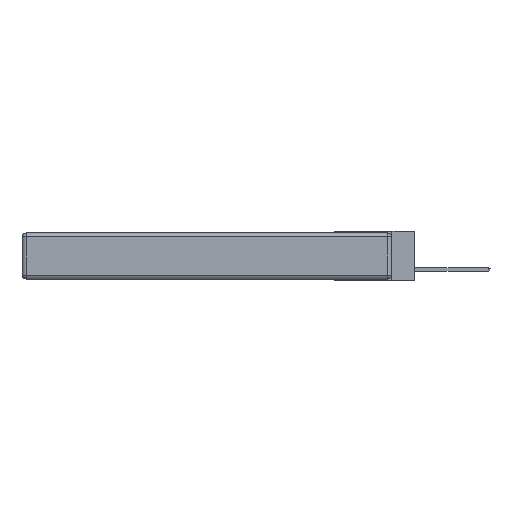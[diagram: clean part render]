
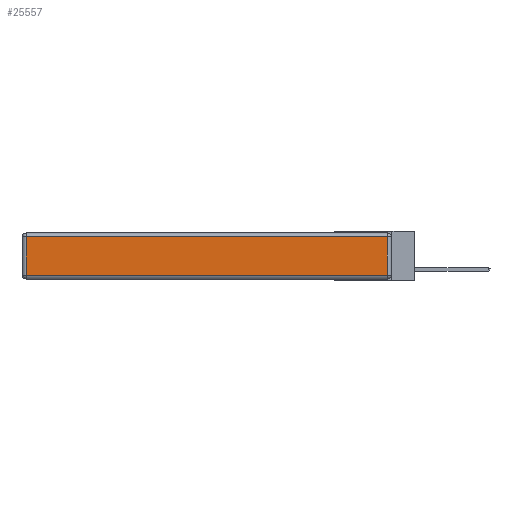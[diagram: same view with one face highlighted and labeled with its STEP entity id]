
A CAD part, left-side view. The second image highlights one B-rep face of the part: STEP entity #25557.
In plain terms, the highlighted planar face has unit normal (-1, 0, 0).
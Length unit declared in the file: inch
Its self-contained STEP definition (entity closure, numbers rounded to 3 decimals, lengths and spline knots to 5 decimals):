
#193 = AXIS2_PLACEMENT_3D ( 'NONE', #6007, #12641, #1880 ) ;
#812 = CARTESIAN_POINT ( 'NONE',  ( 0., 0.03, -0.313 ) ) ;
#1831 = CARTESIAN_POINT ( 'NONE',  ( 0., 0.03, -0.343 ) ) ;
#1880 = DIRECTION ( 'NONE',  ( 0., 0., 1. ) ) ;
#4342 = EDGE_CURVE ( 'NONE', #15104, #18792, #16926, .T. ) ;
#4515 = EDGE_CURVE ( 'NONE', #22478, #13630, #12835, .T. ) ;
#6007 = CARTESIAN_POINT ( 'NONE',  ( 0., 0., -0.343 ) ) ;
#6873 = CARTESIAN_POINT ( 'NONE',  ( 0., 0.03, -0.03 ) ) ;
#6905 = VECTOR ( 'NONE', #7281, 39.37008 ) ;
#7242 = VECTOR ( 'NONE', #12790, 39.37008 ) ;
#7281 = DIRECTION ( 'NONE',  ( 0., 1., 0. ) ) ;
#7695 = FACE_OUTER_BOUND ( 'NONE', #10929, .T. ) ;
#8830 = CARTESIAN_POINT ( 'NONE',  ( 0., 2.72, -0.313 ) ) ;
#10929 = EDGE_LOOP ( 'NONE', ( #24318, #21919, #18268, #20589 ) ) ;
#11512 = DIRECTION ( 'NONE',  ( 0., 0., -1. ) ) ;
#12166 = CARTESIAN_POINT ( 'NONE',  ( 0., 2.75, -0.03 ) ) ;
#12641 = DIRECTION ( 'NONE',  ( -1., 0., 0. ) ) ;
#12747 = LINE ( 'NONE', #17859, #15802 ) ;
#12790 = DIRECTION ( 'NONE',  ( 0., 0., 1. ) ) ;
#12835 = LINE ( 'NONE', #12166, #6905 ) ;
#13112 = CARTESIAN_POINT ( 'NONE',  ( 0., 0., -0.313 ) ) ;
#13630 = VERTEX_POINT ( 'NONE', #17484 ) ;
#14268 = EDGE_CURVE ( 'NONE', #18792, #22478, #27991, .T. ) ;
#15104 = VERTEX_POINT ( 'NONE', #8830 ) ;
#15802 = VECTOR ( 'NONE', #11512, 39.37008 ) ;
#16247 = VECTOR ( 'NONE', #28521, 39.37008 ) ;
#16926 = LINE ( 'NONE', #13112, #16247 ) ;
#17484 = CARTESIAN_POINT ( 'NONE',  ( 0., 2.72, -0.03 ) ) ;
#17859 = CARTESIAN_POINT ( 'NONE',  ( 0., 2.72, -0.343 ) ) ;
#18268 = ORIENTED_EDGE ( 'NONE', *, *, #4515, .T. ) ;
#18792 = VERTEX_POINT ( 'NONE', #812 ) ;
#19354 = PLANE ( 'NONE',  #193 ) ;
#19757 = EDGE_CURVE ( 'NONE', #13630, #15104, #12747, .T. ) ;
#20589 = ORIENTED_EDGE ( 'NONE', *, *, #19757, .T. ) ;
#21919 = ORIENTED_EDGE ( 'NONE', *, *, #14268, .T. ) ;
#22478 = VERTEX_POINT ( 'NONE', #6873 ) ;
#24318 = ORIENTED_EDGE ( 'NONE', *, *, #4342, .T. ) ;
#25557 = ADVANCED_FACE ( 'NONE', ( #7695 ), #19354, .T. ) ;
#27991 = LINE ( 'NONE', #1831, #7242 ) ;
#28521 = DIRECTION ( 'NONE',  ( 0., -1., 0. ) ) ;
